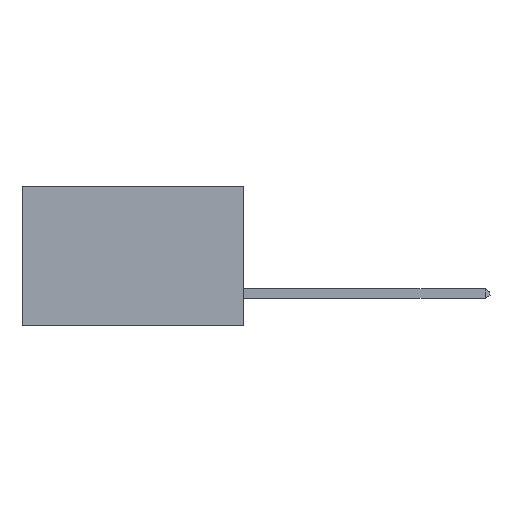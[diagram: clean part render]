
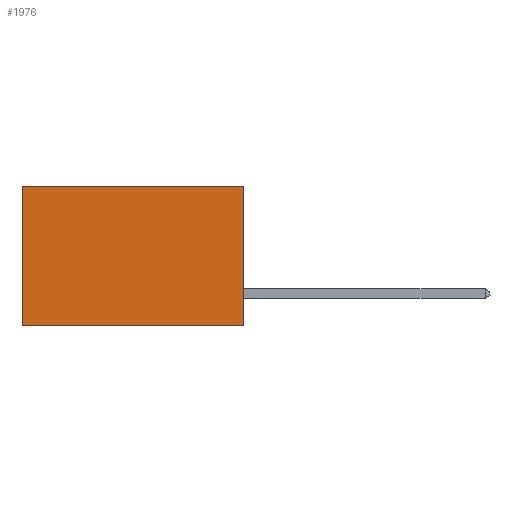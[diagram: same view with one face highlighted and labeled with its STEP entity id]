
A CAD part, left-side view. The second image highlights one B-rep face of the part: STEP entity #1976.
In plain terms, the highlighted planar face has unit normal (-1, 0, 0).
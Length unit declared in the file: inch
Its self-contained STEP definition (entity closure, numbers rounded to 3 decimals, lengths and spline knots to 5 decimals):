
#534 = VERTEX_POINT ( 'NONE', #1941 ) ;
#1206 = LINE ( 'NONE', #7237, #3318 ) ;
#1424 = CARTESIAN_POINT ( 'NONE',  ( 0.277, 0., 0. ) ) ;
#1903 = VERTEX_POINT ( 'NONE', #2026 ) ;
#1923 = DIRECTION ( 'NONE',  ( 0., 1., 0. ) ) ;
#1941 = CARTESIAN_POINT ( 'NONE',  ( 0.277, 0.59, -0.37 ) ) ;
#1976 = ADVANCED_FACE ( 'NONE', ( #5465 ), #5211, .F. ) ;
#1986 = AXIS2_PLACEMENT_3D ( 'NONE', #9633, #9498, #9532 ) ;
#2026 = CARTESIAN_POINT ( 'NONE',  ( 0.277, 0., 0. ) ) ;
#2191 = VERTEX_POINT ( 'NONE', #3982 ) ;
#2378 = LINE ( 'NONE', #1424, #8152 ) ;
#2604 = CARTESIAN_POINT ( 'NONE',  ( 0.277, 0., -0.37 ) ) ;
#3318 = VECTOR ( 'NONE', #7289, 39.37008 ) ;
#3466 = LINE ( 'NONE', #7816, #9080 ) ;
#3529 = EDGE_LOOP ( 'NONE', ( #7986, #8166, #6176, #8784 ) ) ;
#3835 = DIRECTION ( 'NONE',  ( 0., 1., 0. ) ) ;
#3982 = CARTESIAN_POINT ( 'NONE',  ( 0.277, 0.59, 0. ) ) ;
#4609 = EDGE_CURVE ( 'NONE', #7984, #534, #7412, .T. ) ;
#5204 = CARTESIAN_POINT ( 'NONE',  ( 0.277, 0., -0.37 ) ) ;
#5211 = PLANE ( 'NONE',  #1986 ) ;
#5431 = VECTOR ( 'NONE', #3835, 39.37008 ) ;
#5465 = FACE_OUTER_BOUND ( 'NONE', #3529, .T. ) ;
#6176 = ORIENTED_EDGE ( 'NONE', *, *, #6388, .F. ) ;
#6388 = EDGE_CURVE ( 'NONE', #1903, #7984, #3466, .T. ) ;
#7237 = CARTESIAN_POINT ( 'NONE',  ( 0.277, 0.59, -0.37 ) ) ;
#7289 = DIRECTION ( 'NONE',  ( 0., 0., -1. ) ) ;
#7412 = LINE ( 'NONE', #2604, #5431 ) ;
#7816 = CARTESIAN_POINT ( 'NONE',  ( 0.277, 0., -0.37 ) ) ;
#7955 = DIRECTION ( 'NONE',  ( 0., 0., -1. ) ) ;
#7984 = VERTEX_POINT ( 'NONE', #5204 ) ;
#7986 = ORIENTED_EDGE ( 'NONE', *, *, #8806, .T. ) ;
#8103 = EDGE_CURVE ( 'NONE', #1903, #2191, #2378, .T. ) ;
#8152 = VECTOR ( 'NONE', #1923, 39.37008 ) ;
#8166 = ORIENTED_EDGE ( 'NONE', *, *, #4609, .F. ) ;
#8784 = ORIENTED_EDGE ( 'NONE', *, *, #8103, .T. ) ;
#8806 = EDGE_CURVE ( 'NONE', #2191, #534, #1206, .T. ) ;
#9080 = VECTOR ( 'NONE', #7955, 39.37008 ) ;
#9498 = DIRECTION ( 'NONE',  ( 1., 0., 0. ) ) ;
#9532 = DIRECTION ( 'NONE',  ( 0., 0., -1. ) ) ;
#9633 = CARTESIAN_POINT ( 'NONE',  ( 0.277, 0., -0.37 ) ) ;
